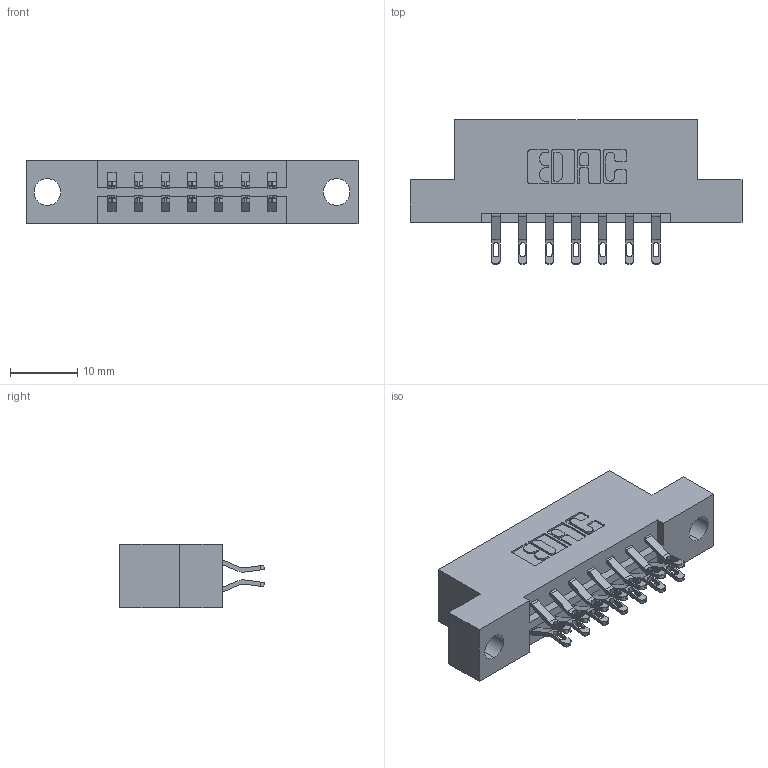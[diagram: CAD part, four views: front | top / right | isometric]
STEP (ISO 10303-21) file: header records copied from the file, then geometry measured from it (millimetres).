
FILE_DESCRIPTION (( 'STEP AP203' ), '1' );
FILE_NAME ('333-014-555-204.STEP', '2018-08-01T02:55:19', ( '' ), ( '' ), 'SwSTEP 2.0', 'SolidWorks 2016', '' );
FILE_SCHEMA (( 'CONFIG_CONTROL_DESIGN' ));
Length unit declared in the file: inch
Products named in the file (3): 333-014-555-204; 333 Part_Flush - .156 Dia - TH; 345-292-001_555 Tail
Assembly tree (15 placements, depth 2):
  333-014-555-204
    333 Part_Flush - .156 Dia - TH
    345-292-001_555 Tail  x14
Bounding box: 49.28 x 21.47 x 9.4 mm (x, y, z)
Volume: 4656.2 mm3; surface area: 5080 mm2
Topology: 15 solids, 15 shells, 926 faces, 2873 edges, 1914 vertices
Faces by surface type: plane 546, cylinder 380
Entity records: 9359 total; most frequent: CARTESIAN_POINT 1628, ORIENTED_EDGE 1534, DIRECTION 1423, EDGE_CURVE 767, LINE 619, VECTOR 619, VERTEX_POINT 510, AXIS2_PLACEMENT_3D 402
